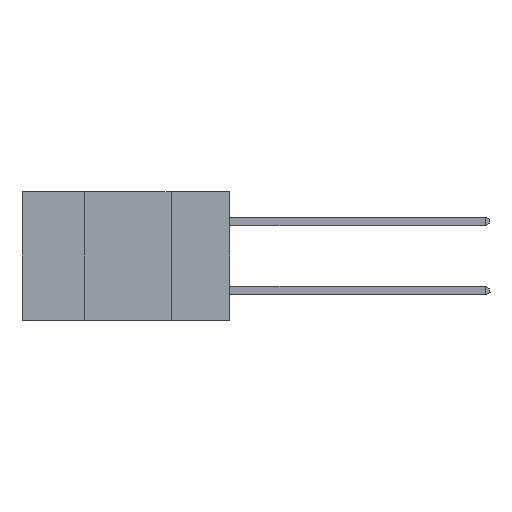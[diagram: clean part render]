
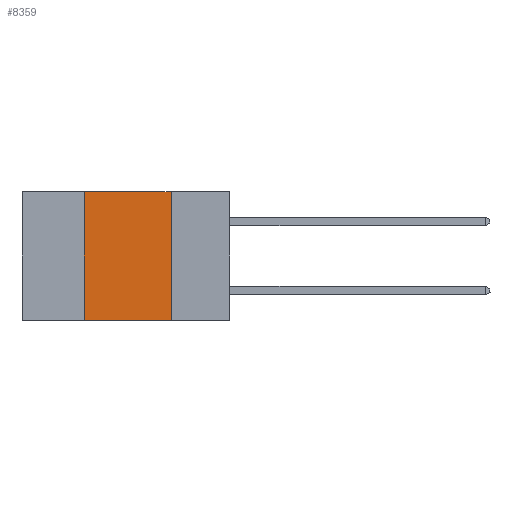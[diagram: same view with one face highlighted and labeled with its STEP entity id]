
A CAD part, left-side view. The second image highlights one B-rep face of the part: STEP entity #8359.
In plain terms, the highlighted planar face has unit normal (-1, 0, 0).
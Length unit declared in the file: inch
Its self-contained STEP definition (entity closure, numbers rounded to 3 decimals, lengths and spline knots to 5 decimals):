
#539 = VERTEX_POINT ( 'NONE', #6866 ) ;
#1058 = LINE ( 'NONE', #5501, #4133 ) ;
#1288 = CARTESIAN_POINT ( 'NONE',  ( 0., 0.17, -0.37 ) ) ;
#1885 = DIRECTION ( 'NONE',  ( 0., 0., 1. ) ) ;
#2012 = DIRECTION ( 'NONE',  ( 0., -1., 0. ) ) ;
#2181 = EDGE_CURVE ( 'NONE', #8665, #8650, #8999, .T. ) ;
#2516 = ORIENTED_EDGE ( 'NONE', *, *, #6613, .T. ) ;
#3087 = DIRECTION ( 'NONE',  ( 0., 0., -1. ) ) ;
#3132 = VERTEX_POINT ( 'NONE', #1288 ) ;
#3194 = CARTESIAN_POINT ( 'NONE',  ( 0., 0.17, 0. ) ) ;
#3274 = LINE ( 'NONE', #5197, #6301 ) ;
#3582 = EDGE_LOOP ( 'NONE', ( #4774, #6307, #9245, #2516 ) ) ;
#4133 = VECTOR ( 'NONE', #3087, 39.37008 ) ;
#4309 = FACE_OUTER_BOUND ( 'NONE', #3582, .T. ) ;
#4318 = EDGE_CURVE ( 'NONE', #539, #8665, #7057, .T. ) ;
#4774 = ORIENTED_EDGE ( 'NONE', *, *, #4911, .F. ) ;
#4911 = EDGE_CURVE ( 'NONE', #8650, #3132, #1058, .T. ) ;
#5091 = CARTESIAN_POINT ( 'NONE',  ( 0., 0.6, 0. ) ) ;
#5197 = CARTESIAN_POINT ( 'NONE',  ( 0., 0.6, -0.37 ) ) ;
#5501 = CARTESIAN_POINT ( 'NONE',  ( 0., 0.17, 0. ) ) ;
#5711 = CARTESIAN_POINT ( 'NONE',  ( 0., 0.6, 0. ) ) ;
#5743 = DIRECTION ( 'NONE',  ( 1., 0., 0. ) ) ;
#5778 = PLANE ( 'NONE',  #6058 ) ;
#5809 = CARTESIAN_POINT ( 'NONE',  ( 0., 0.42, 0. ) ) ;
#6058 = AXIS2_PLACEMENT_3D ( 'NONE', #5711, #5743, #6496 ) ;
#6215 = CARTESIAN_POINT ( 'NONE',  ( 0., 0.42, 0. ) ) ;
#6301 = VECTOR ( 'NONE', #7590, 39.37008 ) ;
#6307 = ORIENTED_EDGE ( 'NONE', *, *, #2181, .F. ) ;
#6496 = DIRECTION ( 'NONE',  ( 0., 0., -1. ) ) ;
#6613 = EDGE_CURVE ( 'NONE', #539, #3132, #3274, .T. ) ;
#6866 = CARTESIAN_POINT ( 'NONE',  ( 0., 0.42, -0.37 ) ) ;
#7057 = LINE ( 'NONE', #5809, #7191 ) ;
#7191 = VECTOR ( 'NONE', #1885, 39.37008 ) ;
#7590 = DIRECTION ( 'NONE',  ( 0., -1., 0. ) ) ;
#8359 = ADVANCED_FACE ( 'NONE', ( #4309 ), #5778, .F. ) ;
#8650 = VERTEX_POINT ( 'NONE', #3194 ) ;
#8665 = VERTEX_POINT ( 'NONE', #6215 ) ;
#8999 = LINE ( 'NONE', #5091, #9471 ) ;
#9245 = ORIENTED_EDGE ( 'NONE', *, *, #4318, .F. ) ;
#9471 = VECTOR ( 'NONE', #2012, 39.37008 ) ;
